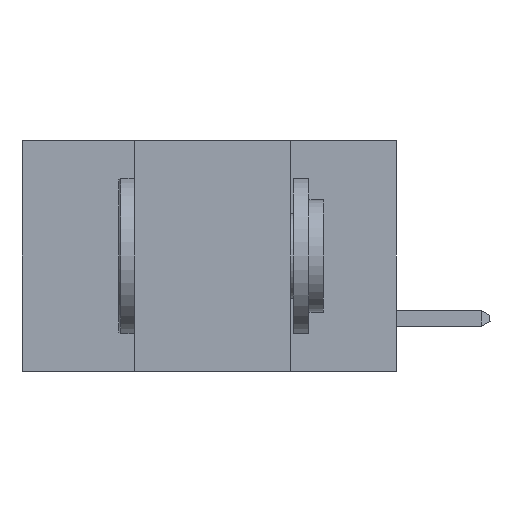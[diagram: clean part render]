
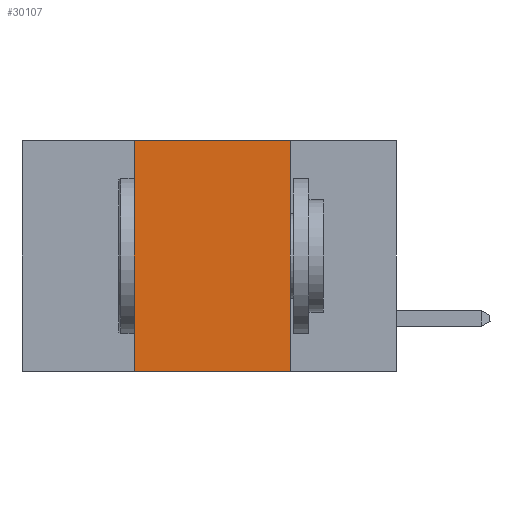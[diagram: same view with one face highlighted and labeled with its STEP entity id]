
A CAD part, left-side view. The second image highlights one B-rep face of the part: STEP entity #30107.
In plain terms, the highlighted planar face has unit normal (-1, 0, 0).
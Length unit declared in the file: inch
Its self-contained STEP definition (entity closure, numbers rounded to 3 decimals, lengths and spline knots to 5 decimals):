
#13 = CARTESIAN_POINT ( 'NONE',  ( 0., 0.17, 0. ) ) ;
#43 = DIRECTION ( 'NONE',  ( 0., 0., -1. ) ) ;
#1267 = ORIENTED_EDGE ( 'NONE', *, *, #16698, .F. ) ;
#1769 = PLANE ( 'NONE',  #25109 ) ;
#3265 = VECTOR ( 'NONE', #21093, 39.37008 ) ;
#3406 = EDGE_CURVE ( 'NONE', #9494, #13578, #11736, .T. ) ;
#4256 = DIRECTION ( 'NONE',  ( 0., 0., -1. ) ) ;
#5001 = EDGE_LOOP ( 'NONE', ( #25700, #1267, #14309, #15071 ) ) ;
#6421 = VECTOR ( 'NONE', #31088, 39.37008 ) ;
#7336 = EDGE_CURVE ( 'NONE', #27431, #11821, #14749, .T. ) ;
#9494 = VERTEX_POINT ( 'NONE', #14592 ) ;
#10504 = CARTESIAN_POINT ( 'NONE',  ( 0., 0.42, 0. ) ) ;
#10655 = CARTESIAN_POINT ( 'NONE',  ( 0., 0.42, -0.37 ) ) ;
#11736 = LINE ( 'NONE', #13, #16689 ) ;
#11821 = VERTEX_POINT ( 'NONE', #19743 ) ;
#12185 = EDGE_CURVE ( 'NONE', #27431, #13578, #13648, .T. ) ;
#13514 = CARTESIAN_POINT ( 'NONE',  ( 0., 0.17, -0.37 ) ) ;
#13578 = VERTEX_POINT ( 'NONE', #13514 ) ;
#13648 = LINE ( 'NONE', #23439, #26587 ) ;
#13659 = DIRECTION ( 'NONE',  ( 0., -1., 0. ) ) ;
#14309 = ORIENTED_EDGE ( 'NONE', *, *, #7336, .F. ) ;
#14592 = CARTESIAN_POINT ( 'NONE',  ( 0., 0.17, 0. ) ) ;
#14749 = LINE ( 'NONE', #10504, #3265 ) ;
#15071 = ORIENTED_EDGE ( 'NONE', *, *, #12185, .T. ) ;
#16367 = CARTESIAN_POINT ( 'NONE',  ( 0., 0.6, 0. ) ) ;
#16661 = CARTESIAN_POINT ( 'NONE',  ( 0., 0.6, 0. ) ) ;
#16689 = VECTOR ( 'NONE', #43, 39.37008 ) ;
#16698 = EDGE_CURVE ( 'NONE', #11821, #9494, #25045, .T. ) ;
#16989 = FACE_OUTER_BOUND ( 'NONE', #5001, .T. ) ;
#18849 = DIRECTION ( 'NONE',  ( 1., 0., 0. ) ) ;
#19743 = CARTESIAN_POINT ( 'NONE',  ( 0., 0.42, 0. ) ) ;
#21093 = DIRECTION ( 'NONE',  ( 0., 0., 1. ) ) ;
#23439 = CARTESIAN_POINT ( 'NONE',  ( 0., 0.6, -0.37 ) ) ;
#25045 = LINE ( 'NONE', #16661, #6421 ) ;
#25109 = AXIS2_PLACEMENT_3D ( 'NONE', #16367, #18849, #4256 ) ;
#25700 = ORIENTED_EDGE ( 'NONE', *, *, #3406, .F. ) ;
#26587 = VECTOR ( 'NONE', #13659, 39.37008 ) ;
#27431 = VERTEX_POINT ( 'NONE', #10655 ) ;
#30107 = ADVANCED_FACE ( 'NONE', ( #16989 ), #1769, .F. ) ;
#31088 = DIRECTION ( 'NONE',  ( 0., -1., 0. ) ) ;
